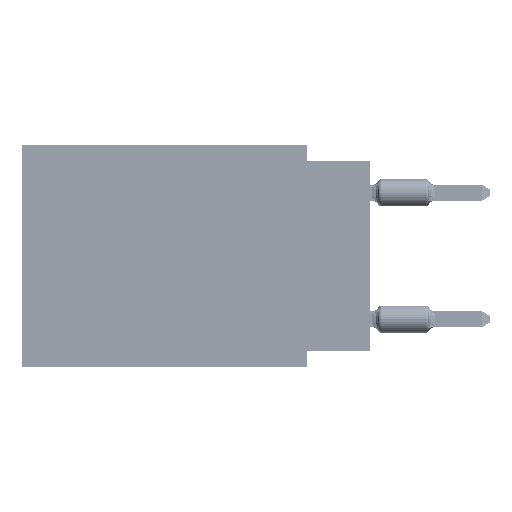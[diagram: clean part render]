
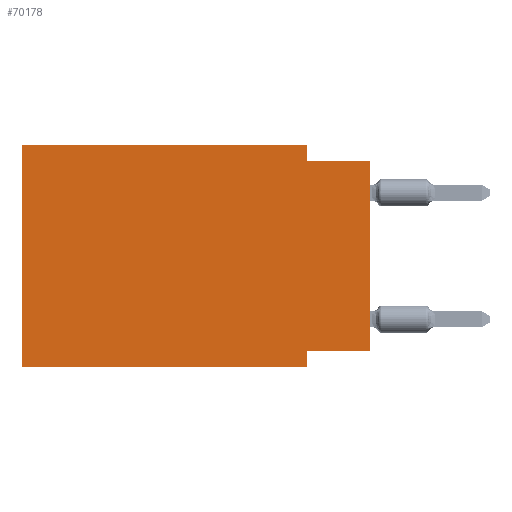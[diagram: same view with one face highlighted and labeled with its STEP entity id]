
A CAD part, left-side view. The second image highlights one B-rep face of the part: STEP entity #70178.
In plain terms, the highlighted planar face has unit normal (-1, 0, 0).
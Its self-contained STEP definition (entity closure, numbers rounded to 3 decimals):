
#2 = CARTESIAN_POINT ( 'NONE',  ( 0., 2.54, -8.255 ) ) ;
#480 = PLANE ( 'NONE',  #58378 ) ;
#1904 = VECTOR ( 'NONE', #3287, 1000. ) ;
#2511 = CARTESIAN_POINT ( 'NONE',  ( 0., 0., -8.255 ) ) ;
#2936 = DIRECTION ( 'NONE',  ( 0., 1., 0. ) ) ;
#3287 = DIRECTION ( 'NONE',  ( 0., 0., -1. ) ) ;
#4037 = ORIENTED_EDGE ( 'NONE', *, *, #10203, .T. ) ;
#7018 = EDGE_CURVE ( 'NONE', #42071, #37269, #29572, .T. ) ;
#7689 = DIRECTION ( 'NONE',  ( 0., -1., 0. ) ) ;
#9874 = CARTESIAN_POINT ( 'NONE',  ( 0., 0., -8.255 ) ) ;
#10203 = EDGE_CURVE ( 'NONE', #85498, #58934, #13279, .T. ) ;
#11179 = DIRECTION ( 'NONE',  ( 0., 0., 1. ) ) ;
#12988 = VECTOR ( 'NONE', #75155, 1000. ) ;
#13207 = VECTOR ( 'NONE', #11179, 1000. ) ;
#13279 = LINE ( 'NONE', #60080, #12988 ) ;
#14771 = LINE ( 'NONE', #2511, #15513 ) ;
#15121 = CARTESIAN_POINT ( 'NONE',  ( 0., 2.54, 0. ) ) ;
#15513 = VECTOR ( 'NONE', #2936, 1000. ) ;
#16796 = VERTEX_POINT ( 'NONE', #62421 ) ;
#18123 = CARTESIAN_POINT ( 'NONE',  ( 0., 2.54, -8.89 ) ) ;
#18217 = EDGE_CURVE ( 'NONE', #51119, #37269, #24253, .T. ) ;
#21438 = ORIENTED_EDGE ( 'NONE', *, *, #48827, .F. ) ;
#22124 = LINE ( 'NONE', #74590, #27017 ) ;
#22146 = DIRECTION ( 'NONE',  ( 0., -1., 0. ) ) ;
#22787 = CARTESIAN_POINT ( 'NONE',  ( 0., 2.54, -8.89 ) ) ;
#24253 = LINE ( 'NONE', #18123, #1904 ) ;
#26064 = LINE ( 'NONE', #52740, #34161 ) ;
#27017 = VECTOR ( 'NONE', #7689, 1000. ) ;
#27369 = LINE ( 'NONE', #15121, #66099 ) ;
#27782 = VECTOR ( 'NONE', #22146, 1000. ) ;
#29572 = LINE ( 'NONE', #55386, #27782 ) ;
#33737 = FACE_OUTER_BOUND ( 'NONE', #56532, .T. ) ;
#34161 = VECTOR ( 'NONE', #78546, 1000. ) ;
#36218 = CARTESIAN_POINT ( 'NONE',  ( 0., 2.54, -0.635 ) ) ;
#37027 = CARTESIAN_POINT ( 'NONE',  ( 0., 13.97, 0. ) ) ;
#37269 = VERTEX_POINT ( 'NONE', #22787 ) ;
#40723 = DIRECTION ( 'NONE',  ( 1., 0., 0. ) ) ;
#42071 = VERTEX_POINT ( 'NONE', #54034 ) ;
#45810 = EDGE_CURVE ( 'NONE', #85498, #51119, #14771, .T. ) ;
#47494 = ORIENTED_EDGE ( 'NONE', *, *, #79463, .F. ) ;
#48349 = ORIENTED_EDGE ( 'NONE', *, *, #18217, .F. ) ;
#48360 = DIRECTION ( 'NONE',  ( 0., 0., -1. ) ) ;
#48827 = EDGE_CURVE ( 'NONE', #16796, #51898, #27369, .T. ) ;
#51119 = VERTEX_POINT ( 'NONE', #2 ) ;
#51898 = VERTEX_POINT ( 'NONE', #36218 ) ;
#52740 = CARTESIAN_POINT ( 'NONE',  ( 0., 13.97, 0. ) ) ;
#54034 = CARTESIAN_POINT ( 'NONE',  ( 0., 13.97, -8.89 ) ) ;
#54795 = EDGE_CURVE ( 'NONE', #59839, #16796, #26064, .T. ) ;
#54929 = EDGE_CURVE ( 'NONE', #51898, #58934, #22124, .T. ) ;
#55386 = CARTESIAN_POINT ( 'NONE',  ( 0., 13.97, -8.89 ) ) ;
#56532 = EDGE_LOOP ( 'NONE', ( #4037, #58216, #21438, #65417, #47494, #85636, #48349, #86392 ) ) ;
#58216 = ORIENTED_EDGE ( 'NONE', *, *, #54929, .F. ) ;
#58378 = AXIS2_PLACEMENT_3D ( 'NONE', #80082, #40723, #81846 ) ;
#58934 = VERTEX_POINT ( 'NONE', #85781 ) ;
#59839 = VERTEX_POINT ( 'NONE', #61307 ) ;
#60080 = CARTESIAN_POINT ( 'NONE',  ( 0., 0., 0. ) ) ;
#61307 = CARTESIAN_POINT ( 'NONE',  ( 0., 13.97, 0. ) ) ;
#62421 = CARTESIAN_POINT ( 'NONE',  ( 0., 2.54, 0. ) ) ;
#65417 = ORIENTED_EDGE ( 'NONE', *, *, #54795, .F. ) ;
#66099 = VECTOR ( 'NONE', #48360, 1000. ) ;
#70178 = ADVANCED_FACE ( 'NONE', ( #33737 ), #480, .F. ) ;
#74590 = CARTESIAN_POINT ( 'NONE',  ( 0., 0., -0.635 ) ) ;
#75155 = DIRECTION ( 'NONE',  ( 0., 0., 1. ) ) ;
#78546 = DIRECTION ( 'NONE',  ( 0., -1., 0. ) ) ;
#79463 = EDGE_CURVE ( 'NONE', #42071, #59839, #83389, .T. ) ;
#80082 = CARTESIAN_POINT ( 'NONE',  ( 0., 13.97, 0. ) ) ;
#81846 = DIRECTION ( 'NONE',  ( 0., 0., -1. ) ) ;
#83389 = LINE ( 'NONE', #37027, #13207 ) ;
#85498 = VERTEX_POINT ( 'NONE', #9874 ) ;
#85636 = ORIENTED_EDGE ( 'NONE', *, *, #7018, .T. ) ;
#85781 = CARTESIAN_POINT ( 'NONE',  ( 0., 0., -0.635 ) ) ;
#86392 = ORIENTED_EDGE ( 'NONE', *, *, #45810, .F. ) ;
